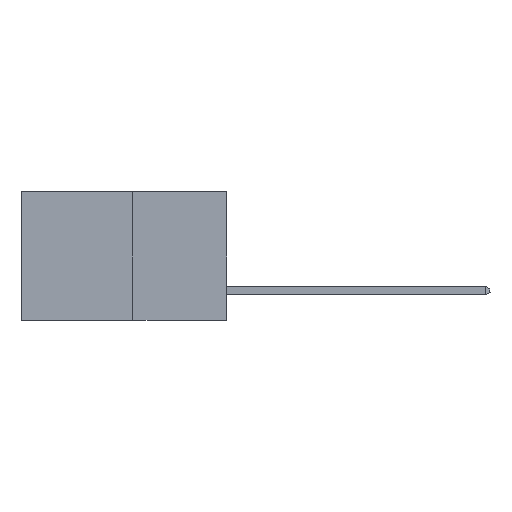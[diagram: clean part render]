
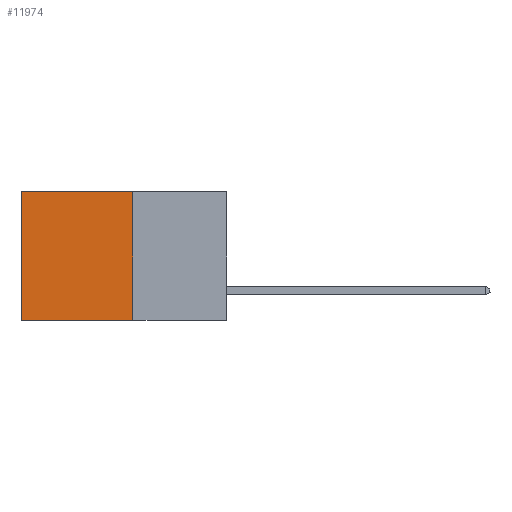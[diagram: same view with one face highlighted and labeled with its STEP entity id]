
A CAD part, left-side view. The second image highlights one B-rep face of the part: STEP entity #11974.
In plain terms, the highlighted planar face has unit normal (-1, 0, 0).
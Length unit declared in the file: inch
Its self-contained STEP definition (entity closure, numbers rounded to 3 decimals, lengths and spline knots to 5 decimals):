
#63 = CARTESIAN_POINT ( 'NONE',  ( 0.277, 0.59, -0.37 ) ) ;
#1132 = VERTEX_POINT ( 'NONE', #12813 ) ;
#1284 = DIRECTION ( 'NONE',  ( 0., 0., -1. ) ) ;
#1565 = VECTOR ( 'NONE', #15330, 39.37008 ) ;
#2772 = EDGE_CURVE ( 'NONE', #1132, #13493, #7417, .T. ) ;
#2785 = CARTESIAN_POINT ( 'NONE',  ( 0.277, 0.27, -0.37 ) ) ;
#2857 = LINE ( 'NONE', #12268, #5826 ) ;
#3569 = EDGE_LOOP ( 'NONE', ( #7691, #8077, #12087, #8668 ) ) ;
#4285 = VECTOR ( 'NONE', #9043, 39.37008 ) ;
#4337 = DIRECTION ( 'NONE',  ( 1., 0., 0. ) ) ;
#5826 = VECTOR ( 'NONE', #13519, 39.37008 ) ;
#5947 = VERTEX_POINT ( 'NONE', #11358 ) ;
#7417 = LINE ( 'NONE', #9686, #1565 ) ;
#7586 = LINE ( 'NONE', #2785, #4285 ) ;
#7647 = FACE_OUTER_BOUND ( 'NONE', #3569, .T. ) ;
#7691 = ORIENTED_EDGE ( 'NONE', *, *, #12208, .T. ) ;
#7998 = AXIS2_PLACEMENT_3D ( 'NONE', #10488, #4337, #12948 ) ;
#8077 = ORIENTED_EDGE ( 'NONE', *, *, #2772, .F. ) ;
#8438 = EDGE_CURVE ( 'NONE', #13860, #5947, #2857, .T. ) ;
#8668 = ORIENTED_EDGE ( 'NONE', *, *, #8438, .T. ) ;
#9043 = DIRECTION ( 'NONE',  ( 0., 0., -1. ) ) ;
#9686 = CARTESIAN_POINT ( 'NONE',  ( 0.277, 0.27, -0.37 ) ) ;
#10488 = CARTESIAN_POINT ( 'NONE',  ( 0.277, 0.27, -0.37 ) ) ;
#10544 = CARTESIAN_POINT ( 'NONE',  ( 0.277, 0.27, 0. ) ) ;
#11137 = CARTESIAN_POINT ( 'NONE',  ( 0.277, 0.59, -0.37 ) ) ;
#11358 = CARTESIAN_POINT ( 'NONE',  ( 0.277, 0.59, 0. ) ) ;
#11974 = ADVANCED_FACE ( 'NONE', ( #7647 ), #12893, .F. ) ;
#12087 = ORIENTED_EDGE ( 'NONE', *, *, #13676, .F. ) ;
#12208 = EDGE_CURVE ( 'NONE', #5947, #13493, #14366, .T. ) ;
#12268 = CARTESIAN_POINT ( 'NONE',  ( 0.277, 0.27, 0. ) ) ;
#12813 = CARTESIAN_POINT ( 'NONE',  ( 0.277, 0.27, -0.37 ) ) ;
#12893 = PLANE ( 'NONE',  #7998 ) ;
#12948 = DIRECTION ( 'NONE',  ( 0., 0., -1. ) ) ;
#13493 = VERTEX_POINT ( 'NONE', #11137 ) ;
#13519 = DIRECTION ( 'NONE',  ( 0., 1., 0. ) ) ;
#13581 = VECTOR ( 'NONE', #1284, 39.37008 ) ;
#13676 = EDGE_CURVE ( 'NONE', #13860, #1132, #7586, .T. ) ;
#13860 = VERTEX_POINT ( 'NONE', #10544 ) ;
#14366 = LINE ( 'NONE', #63, #13581 ) ;
#15330 = DIRECTION ( 'NONE',  ( 0., 1., 0. ) ) ;
